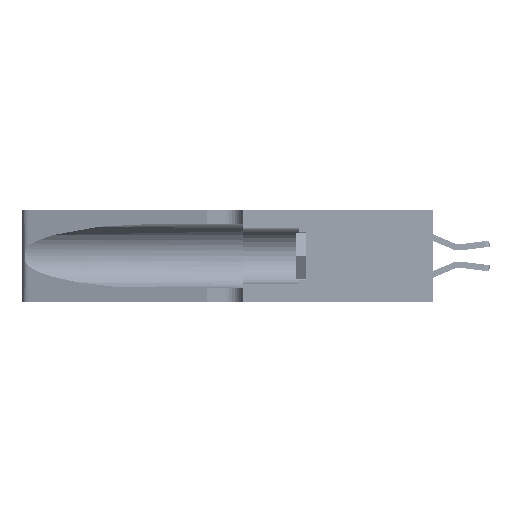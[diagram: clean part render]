
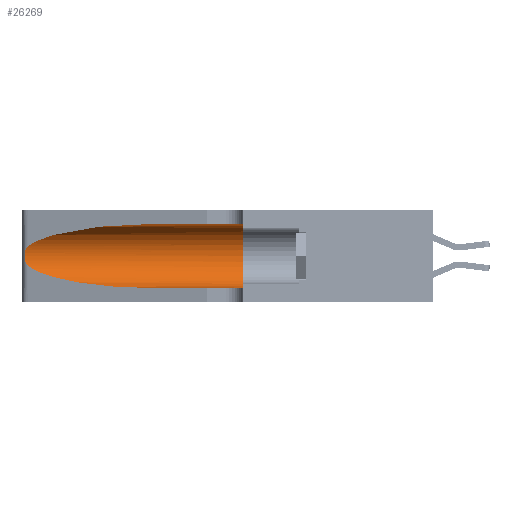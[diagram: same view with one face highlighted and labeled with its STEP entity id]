
A CAD part, left-side view. The second image highlights one B-rep face of the part: STEP entity #26269.
In plain terms, the highlighted cylindrical face has radius 3.308 mm (diameter 6.617 mm), a partial arc.
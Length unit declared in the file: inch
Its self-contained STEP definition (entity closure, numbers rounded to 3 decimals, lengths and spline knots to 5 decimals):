
#127 = CARTESIAN_POINT ( 'NONE',  ( 0.1305, 1.61858, 0.185 ) ) ;
#522 = FACE_OUTER_BOUND ( 'NONE', #38306, .T. ) ;
#3064 = VERTEX_POINT ( 'NONE', #47345 ) ;
#4681 = CARTESIAN_POINT ( 'NONE',  ( 0.25487, 1.22718, 0.22369 ) ) ;
#5175 = CARTESIAN_POINT ( 'NONE',  ( 0.2373, 1.15595, 0.28018 ) ) ;
#7106 = EDGE_CURVE ( 'NONE', #33010, #38619, #31035, .T. ) ;
#7373 = CARTESIAN_POINT ( 'NONE',  ( 0.1305, 1.61858, 0.31525 ) ) ;
#8369 = LINE ( 'NONE', #7373, #13078 ) ;
#8805 = CARTESIAN_POINT ( 'NONE',  ( 0.1305, 0.72297, 0.05475 ) ) ;
#9894 = CARTESIAN_POINT ( 'NONE',  ( 0.25856, 1.23593, 0.16098 ) ) ;
#10050 = CARTESIAN_POINT ( 'NONE',  ( 0.25854, 1.2359, 0.20912 ) ) ;
#10395 = CARTESIAN_POINT ( 'NONE',  ( 0.1305, 0.35, 0.05475 ) ) ;
#11203 = AXIS2_PLACEMENT_3D ( 'NONE', #127, #19695, #26851 ) ;
#11481 = CARTESIAN_POINT ( 'NONE',  ( 0.2373, 1.15595, 0.08982 ) ) ;
#12432 = CARTESIAN_POINT ( 'NONE',  ( 0.18966, 0.96281, 0.31525 ) ) ;
#13078 = VECTOR ( 'NONE', #14792, 39.37008 ) ;
#13414 = CIRCLE ( 'NONE', #43067, 0.13025 ) ;
#13801 = ORIENTED_EDGE ( 'NONE', *, *, #38596, .F. ) ;
#13993 = CARTESIAN_POINT ( 'NONE',  ( 0.25789, 1.23486, 0.15765 ) ) ;
#14792 = DIRECTION ( 'NONE',  ( 0., -1., 0. ) ) ;
#15105 = CARTESIAN_POINT ( 'NONE',  ( 0.1305, 0.72297, 0.05475 ) ) ;
#15685 = ORIENTED_EDGE ( 'NONE', *, *, #7106, .T. ) ;
#17344 = CARTESIAN_POINT ( 'NONE',  ( 0.25487, 1.22718, 0.22369 ) ) ;
#18044 = DIRECTION ( 'NONE',  ( 0., 0., 1. ) ) ;
#18601 = CARTESIAN_POINT ( 'NONE',  ( 0.18966, 0.96281, 0.05475 ) ) ;
#19133 =( BOUNDED_CURVE ( )  B_SPLINE_CURVE ( 3, ( #31221, #12432, #5175, #4681 ),
 .UNSPECIFIED., .F., .F. ) 
 B_SPLINE_CURVE_WITH_KNOTS ( ( 4, 4 ),
 ( 1.5708, 2.84003 ),
 .UNSPECIFIED. ) 
 CURVE ( )  GEOMETRIC_REPRESENTATION_ITEM ( )  RATIONAL_B_SPLINE_CURVE ( ( 1., 0.87, 0.87, 1. ) ) 
 REPRESENTATION_ITEM ( '' )  );
#19695 = DIRECTION ( 'NONE',  ( 0., -1., 0. ) ) ;
#20988 = CARTESIAN_POINT ( 'NONE',  ( 0.25787, 1.23484, 0.2124 ) ) ;
#21173 = EDGE_CURVE ( 'NONE', #38266, #45209, #30781, .T. ) ;
#21291 = CYLINDRICAL_SURFACE ( 'NONE', #11203, 0.13025 ) ;
#21535 = CARTESIAN_POINT ( 'NONE',  ( 0.25487, 1.22718, 0.14631 ) ) ;
#25416 = EDGE_CURVE ( 'NONE', #44345, #3064, #8369, .T. ) ;
#26269 = ADVANCED_FACE ( 'NONE', ( #522 ), #21291, .F. ) ;
#26851 = DIRECTION ( 'NONE',  ( 0., 0., -1. ) ) ;
#26869 = CARTESIAN_POINT ( 'NONE',  ( 0.25487, 1.22718, 0.22369 ) ) ;
#28185 = EDGE_CURVE ( 'NONE', #38619, #38266, #33186, .T. ) ;
#28805 = CARTESIAN_POINT ( 'NONE',  ( 0.25555, 1.22994, 0.2215 ) ) ;
#28865 = DIRECTION ( 'NONE',  ( 0., 1., 0. ) ) ;
#29333 = ORIENTED_EDGE ( 'NONE', *, *, #21173, .T. ) ;
#30781 = LINE ( 'NONE', #42469, #48668 ) ;
#31035 = B_SPLINE_CURVE_WITH_KNOTS ( 'NONE', 3,
 ( #17344, #28805, #43952, #20988, #10050, #32807, #47811, #43790, #40627, #9894, #13993, #44445, #40147, #40468 ),
 .UNSPECIFIED., .F., .F.,
 ( 4, 2, 2, 2, 2, 2, 4 ),
 ( 0., 0.00027, 0.00053, 0.00107, 0.0016, 0.00187, 0.00214 ),
 .UNSPECIFIED. ) ;
#31221 = CARTESIAN_POINT ( 'NONE',  ( 0.1305, 0.72297, 0.31525 ) ) ;
#31342 = ORIENTED_EDGE ( 'NONE', *, *, #25416, .F. ) ;
#32807 = CARTESIAN_POINT ( 'NONE',  ( 0.26018, 1.23835, 0.19895 ) ) ;
#33010 = VERTEX_POINT ( 'NONE', #26869 ) ;
#33186 =( BOUNDED_CURVE ( )  B_SPLINE_CURVE ( 3, ( #33892, #11481, #18601, #15105 ),
 .UNSPECIFIED., .F., .F. ) 
 B_SPLINE_CURVE_WITH_KNOTS ( ( 4, 4 ),
 ( 3.44316, 4.71239 ),
 .UNSPECIFIED. ) 
 CURVE ( )  GEOMETRIC_REPRESENTATION_ITEM ( )  RATIONAL_B_SPLINE_CURVE ( ( 1., 0.87, 0.87, 1. ) ) 
 REPRESENTATION_ITEM ( '' )  );
#33892 = CARTESIAN_POINT ( 'NONE',  ( 0.25487, 1.22718, 0.14631 ) ) ;
#35537 = CARTESIAN_POINT ( 'NONE',  ( 0.1305, 0.72297, 0.31525 ) ) ;
#36544 = ORIENTED_EDGE ( 'NONE', *, *, #46213, .T. ) ;
#38266 = VERTEX_POINT ( 'NONE', #8805 ) ;
#38306 = EDGE_LOOP ( 'NONE', ( #36544, #15685, #48008, #29333, #13801, #31342 ) ) ;
#38596 = EDGE_CURVE ( 'NONE', #3064, #45209, #13414, .T. ) ;
#38619 = VERTEX_POINT ( 'NONE', #21535 ) ;
#40147 = CARTESIAN_POINT ( 'NONE',  ( 0.25555, 1.22993, 0.14849 ) ) ;
#40468 = CARTESIAN_POINT ( 'NONE',  ( 0.25487, 1.22718, 0.14631 ) ) ;
#40573 = DIRECTION ( 'NONE',  ( 0., -1., 0. ) ) ;
#40627 = CARTESIAN_POINT ( 'NONE',  ( 0.26017, 1.23833, 0.17102 ) ) ;
#42469 = CARTESIAN_POINT ( 'NONE',  ( 0.1305, 1.61858, 0.05475 ) ) ;
#43067 = AXIS2_PLACEMENT_3D ( 'NONE', #48509, #28865, #18044 ) ;
#43790 = CARTESIAN_POINT ( 'NONE',  ( 0.26075, 1.23896, 0.178 ) ) ;
#43952 = CARTESIAN_POINT ( 'NONE',  ( 0.25639, 1.23184, 0.21858 ) ) ;
#44345 = VERTEX_POINT ( 'NONE', #35537 ) ;
#44445 = CARTESIAN_POINT ( 'NONE',  ( 0.25639, 1.23186, 0.15144 ) ) ;
#45209 = VERTEX_POINT ( 'NONE', #10395 ) ;
#46213 = EDGE_CURVE ( 'NONE', #44345, #33010, #19133, .T. ) ;
#47345 = CARTESIAN_POINT ( 'NONE',  ( 0.1305, 0.35, 0.31525 ) ) ;
#47811 = CARTESIAN_POINT ( 'NONE',  ( 0.26075, 1.23896, 0.19203 ) ) ;
#48008 = ORIENTED_EDGE ( 'NONE', *, *, #28185, .T. ) ;
#48509 = CARTESIAN_POINT ( 'NONE',  ( 0.1305, 0.35, 0.185 ) ) ;
#48668 = VECTOR ( 'NONE', #40573, 39.37008 ) ;
